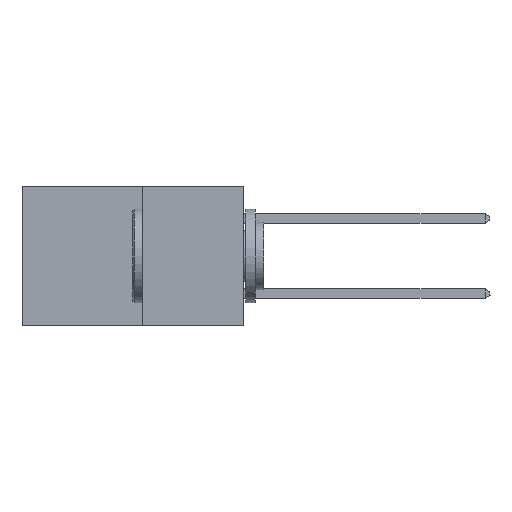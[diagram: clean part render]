
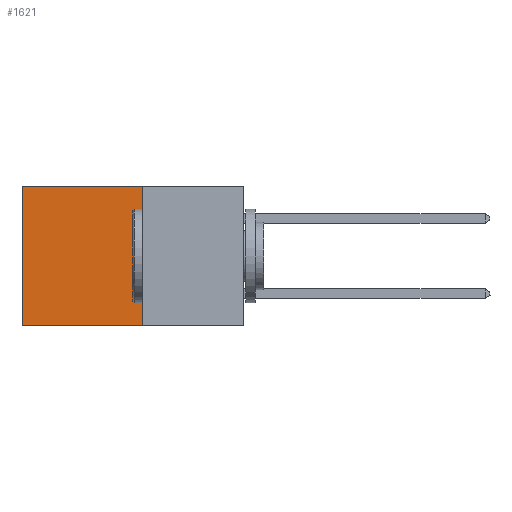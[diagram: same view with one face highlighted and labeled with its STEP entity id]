
A CAD part, left-side view. The second image highlights one B-rep face of the part: STEP entity #1621.
In plain terms, the highlighted planar face has unit normal (-1, 0, 0).
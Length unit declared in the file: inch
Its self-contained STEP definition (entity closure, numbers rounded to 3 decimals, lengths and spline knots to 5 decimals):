
#16 = CARTESIAN_POINT ( 'NONE',  ( 0.277, 0.27, -0.37 ) ) ;
#85 = DIRECTION ( 'NONE',  ( 0., 0., -1. ) ) ;
#199 = EDGE_CURVE ( 'NONE', #4605, #6164, #8762, .T. ) ;
#572 = EDGE_CURVE ( 'NONE', #4471, #6164, #9152, .T. ) ;
#664 = DIRECTION ( 'NONE',  ( 0., 0., -1. ) ) ;
#1060 = EDGE_CURVE ( 'NONE', #6894, #4471, #6833, .T. ) ;
#1173 = FACE_OUTER_BOUND ( 'NONE', #4981, .T. ) ;
#1585 = DIRECTION ( 'NONE',  ( 0., 1., 0. ) ) ;
#1621 = ADVANCED_FACE ( 'NONE', ( #1173 ), #3519, .F. ) ;
#1683 = ORIENTED_EDGE ( 'NONE', *, *, #199, .T. ) ;
#1820 = ORIENTED_EDGE ( 'NONE', *, *, #572, .F. ) ;
#1892 = CARTESIAN_POINT ( 'NONE',  ( 0.277, 0.27, 0. ) ) ;
#1990 = CARTESIAN_POINT ( 'NONE',  ( 0.277, 0.27, 0. ) ) ;
#2238 = ORIENTED_EDGE ( 'NONE', *, *, #1060, .F. ) ;
#2431 = ORIENTED_EDGE ( 'NONE', *, *, #3675, .T. ) ;
#3519 = PLANE ( 'NONE',  #7512 ) ;
#3523 = CARTESIAN_POINT ( 'NONE',  ( 0.277, 0.27, -0.37 ) ) ;
#3675 = EDGE_CURVE ( 'NONE', #6894, #4605, #5247, .T. ) ;
#3800 = CARTESIAN_POINT ( 'NONE',  ( 0.277, 0.59, -0.37 ) ) ;
#4471 = VERTEX_POINT ( 'NONE', #3523 ) ;
#4605 = VERTEX_POINT ( 'NONE', #5831 ) ;
#4846 = VECTOR ( 'NONE', #85, 39.37008 ) ;
#4981 = EDGE_LOOP ( 'NONE', ( #1683, #1820, #2238, #2431 ) ) ;
#5020 = VECTOR ( 'NONE', #6690, 39.37008 ) ;
#5247 = LINE ( 'NONE', #1892, #5020 ) ;
#5544 = DIRECTION ( 'NONE',  ( 1., 0., 0. ) ) ;
#5831 = CARTESIAN_POINT ( 'NONE',  ( 0.277, 0.59, 0. ) ) ;
#6164 = VERTEX_POINT ( 'NONE', #9871 ) ;
#6690 = DIRECTION ( 'NONE',  ( 0., 1., 0. ) ) ;
#6833 = LINE ( 'NONE', #7469, #8452 ) ;
#6894 = VERTEX_POINT ( 'NONE', #1990 ) ;
#7174 = VECTOR ( 'NONE', #1585, 39.37008 ) ;
#7469 = CARTESIAN_POINT ( 'NONE',  ( 0.277, 0.27, -0.37 ) ) ;
#7512 = AXIS2_PLACEMENT_3D ( 'NONE', #8286, #5544, #8279 ) ;
#8279 = DIRECTION ( 'NONE',  ( 0., 0., -1. ) ) ;
#8286 = CARTESIAN_POINT ( 'NONE',  ( 0.277, 0.27, -0.37 ) ) ;
#8452 = VECTOR ( 'NONE', #664, 39.37008 ) ;
#8762 = LINE ( 'NONE', #3800, #4846 ) ;
#9152 = LINE ( 'NONE', #16, #7174 ) ;
#9871 = CARTESIAN_POINT ( 'NONE',  ( 0.277, 0.59, -0.37 ) ) ;
